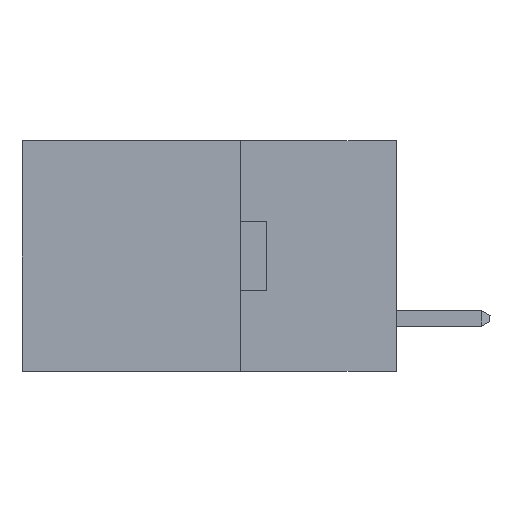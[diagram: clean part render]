
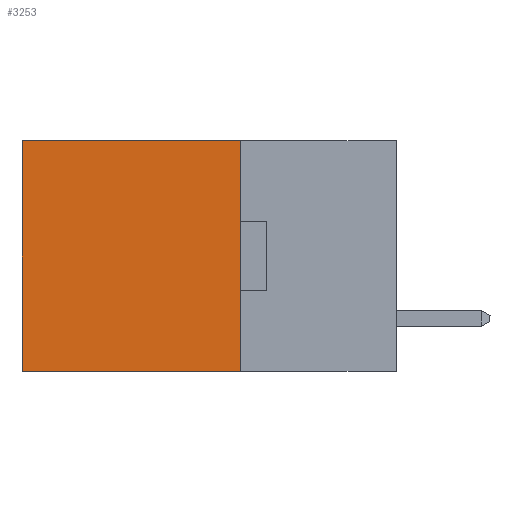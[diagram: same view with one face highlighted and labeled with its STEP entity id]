
A CAD part, left-side view. The second image highlights one B-rep face of the part: STEP entity #3253.
In plain terms, the highlighted planar face has unit normal (-1, 0, 0).
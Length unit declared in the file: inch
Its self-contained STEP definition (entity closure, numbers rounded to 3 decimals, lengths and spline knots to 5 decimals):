
#280 = CARTESIAN_POINT ( 'NONE',  ( 0.2615, 0.6, -0.37 ) ) ;
#305 = EDGE_CURVE ( 'NONE', #14622, #10977, #20227, .T. ) ;
#1231 = VECTOR ( 'NONE', #17837, 39.37008 ) ;
#2494 = CARTESIAN_POINT ( 'NONE',  ( 0.2615, 0.25, -0.37 ) ) ;
#3253 = ADVANCED_FACE ( 'NONE', ( #12562 ), #8552, .F. ) ;
#3875 = VECTOR ( 'NONE', #19740, 39.37008 ) ;
#4740 = CARTESIAN_POINT ( 'NONE',  ( 0.2615, 0.25, -0.37 ) ) ;
#5888 = EDGE_CURVE ( 'NONE', #11569, #16386, #7322, .T. ) ;
#6185 = AXIS2_PLACEMENT_3D ( 'NONE', #8393, #8385, #8354 ) ;
#7206 = ORIENTED_EDGE ( 'NONE', *, *, #11251, .T. ) ;
#7322 = LINE ( 'NONE', #17332, #1231 ) ;
#7332 = VECTOR ( 'NONE', #9474, 39.37008 ) ;
#7415 = CARTESIAN_POINT ( 'NONE',  ( 0.2615, 0.25, -0.37 ) ) ;
#8354 = DIRECTION ( 'NONE',  ( 0., 0., -1. ) ) ;
#8385 = DIRECTION ( 'NONE',  ( 1., 0., 0. ) ) ;
#8393 = CARTESIAN_POINT ( 'NONE',  ( 0.2615, 0.25, -0.37 ) ) ;
#8552 = PLANE ( 'NONE',  #6185 ) ;
#9474 = DIRECTION ( 'NONE',  ( 0., 1., 0. ) ) ;
#9969 = LINE ( 'NONE', #11586, #3875 ) ;
#10592 = CARTESIAN_POINT ( 'NONE',  ( 0.2615, 0.6, 0. ) ) ;
#10977 = VERTEX_POINT ( 'NONE', #2494 ) ;
#11251 = EDGE_CURVE ( 'NONE', #14622, #11569, #9969, .T. ) ;
#11392 = EDGE_LOOP ( 'NONE', ( #26189, #25007, #25901, #7206 ) ) ;
#11569 = VERTEX_POINT ( 'NONE', #10592 ) ;
#11586 = CARTESIAN_POINT ( 'NONE',  ( 0.2615, 0.25, 0. ) ) ;
#12319 = DIRECTION ( 'NONE',  ( 0., 0., -1. ) ) ;
#12562 = FACE_OUTER_BOUND ( 'NONE', #11392, .T. ) ;
#12784 = LINE ( 'NONE', #7415, #7332 ) ;
#14622 = VERTEX_POINT ( 'NONE', #25123 ) ;
#14759 = VECTOR ( 'NONE', #12319, 39.37008 ) ;
#16386 = VERTEX_POINT ( 'NONE', #280 ) ;
#17332 = CARTESIAN_POINT ( 'NONE',  ( 0.2615, 0.6, -0.37 ) ) ;
#17837 = DIRECTION ( 'NONE',  ( 0., 0., -1. ) ) ;
#18937 = EDGE_CURVE ( 'NONE', #10977, #16386, #12784, .T. ) ;
#19740 = DIRECTION ( 'NONE',  ( 0., 1., 0. ) ) ;
#20227 = LINE ( 'NONE', #4740, #14759 ) ;
#25007 = ORIENTED_EDGE ( 'NONE', *, *, #18937, .F. ) ;
#25123 = CARTESIAN_POINT ( 'NONE',  ( 0.2615, 0.25, 0. ) ) ;
#25901 = ORIENTED_EDGE ( 'NONE', *, *, #305, .F. ) ;
#26189 = ORIENTED_EDGE ( 'NONE', *, *, #5888, .T. ) ;
